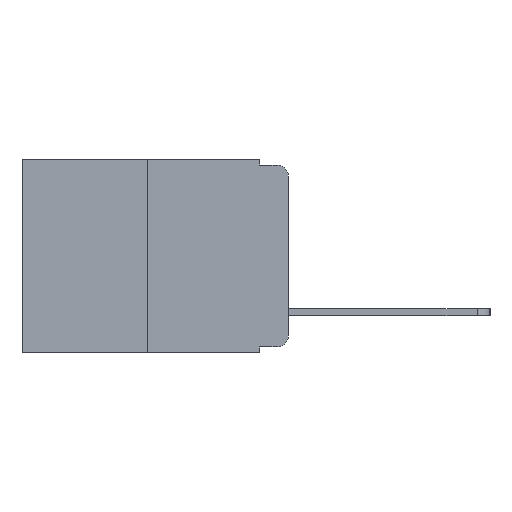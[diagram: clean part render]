
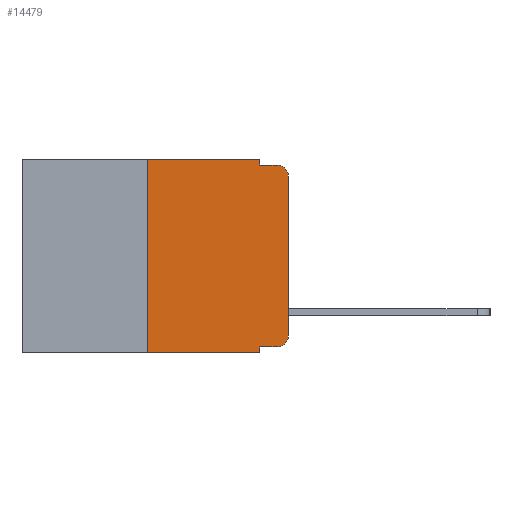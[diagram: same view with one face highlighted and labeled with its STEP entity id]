
A CAD part, left-side view. The second image highlights one B-rep face of the part: STEP entity #14479.
In plain terms, the highlighted planar face has unit normal (-1, 0, 0).
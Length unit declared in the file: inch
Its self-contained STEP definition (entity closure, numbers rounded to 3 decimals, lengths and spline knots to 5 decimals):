
#129 = CARTESIAN_POINT ( 'NONE',  ( 0., 0.02, -0.333 ) ) ;
#312 = CARTESIAN_POINT ( 'NONE',  ( 0., 0.051, 0. ) ) ;
#327 = CARTESIAN_POINT ( 'NONE',  ( 0., 0.02, -0.03 ) ) ;
#511 = FACE_OUTER_BOUND ( 'NONE', #15058, .T. ) ;
#1248 = ORIENTED_EDGE ( 'NONE', *, *, #13304, .T. ) ;
#1250 = DIRECTION ( 'NONE',  ( 0., 0., -1. ) ) ;
#1669 = LINE ( 'NONE', #10075, #18219 ) ;
#2333 = DIRECTION ( 'NONE',  ( 0., 0., -1. ) ) ;
#2387 = VECTOR ( 'NONE', #7106, 39.37008 ) ;
#2648 = CARTESIAN_POINT ( 'NONE',  ( 0., 0.051, 0. ) ) ;
#2941 = EDGE_CURVE ( 'NONE', #19305, #21995, #11428, .T. ) ;
#2993 = LINE ( 'NONE', #20361, #2387 ) ;
#3314 = CARTESIAN_POINT ( 'NONE',  ( 0., 0.051, 0. ) ) ;
#3484 = DIRECTION ( 'NONE',  ( 0., 0., -1. ) ) ;
#3697 = EDGE_CURVE ( 'NONE', #3745, #8694, #10330, .T. ) ;
#3732 = VERTEX_POINT ( 'NONE', #7058 ) ;
#3745 = VERTEX_POINT ( 'NONE', #2648 ) ;
#4067 = CARTESIAN_POINT ( 'NONE',  ( 0., 0.25, -0.343 ) ) ;
#4277 = ORIENTED_EDGE ( 'NONE', *, *, #2941, .T. ) ;
#4304 = VECTOR ( 'NONE', #4906, 39.37008 ) ;
#4624 = ORIENTED_EDGE ( 'NONE', *, *, #7235, .T. ) ;
#4906 = DIRECTION ( 'NONE',  ( 0., -1., 0. ) ) ;
#5001 = DIRECTION ( 'NONE',  ( 0., 0., 1. ) ) ;
#5037 = ORIENTED_EDGE ( 'NONE', *, *, #8382, .T. ) ;
#5169 = ORIENTED_EDGE ( 'NONE', *, *, #20959, .F. ) ;
#5822 = VECTOR ( 'NONE', #3484, 39.37008 ) ;
#5860 = AXIS2_PLACEMENT_3D ( 'NONE', #10078, #11786, #1250 ) ;
#6322 = CARTESIAN_POINT ( 'NONE',  ( 0., 0., -0.313 ) ) ;
#6383 = CARTESIAN_POINT ( 'NONE',  ( 0., 0.051, -0.333 ) ) ;
#6390 = VERTEX_POINT ( 'NONE', #15175 ) ;
#6841 = VERTEX_POINT ( 'NONE', #6383 ) ;
#7058 = CARTESIAN_POINT ( 'NONE',  ( 0., 0.051, -0.343 ) ) ;
#7106 = DIRECTION ( 'NONE',  ( 0., -1., 0. ) ) ;
#7235 = EDGE_CURVE ( 'NONE', #21995, #15967, #21006, .T. ) ;
#8260 = EDGE_CURVE ( 'NONE', #21812, #3732, #20229, .T. ) ;
#8339 = LINE ( 'NONE', #12148, #16635 ) ;
#8382 = EDGE_CURVE ( 'NONE', #15967, #11185, #14354, .T. ) ;
#8426 = PLANE ( 'NONE',  #5860 ) ;
#8650 = ORIENTED_EDGE ( 'NONE', *, *, #3697, .F. ) ;
#8690 = LINE ( 'NONE', #312, #16982 ) ;
#8694 = VERTEX_POINT ( 'NONE', #11718 ) ;
#8819 = EDGE_CURVE ( 'NONE', #6390, #3745, #8339, .T. ) ;
#9137 = ORIENTED_EDGE ( 'NONE', *, *, #8260, .T. ) ;
#10075 = CARTESIAN_POINT ( 'NONE',  ( 0., 0.25, 0. ) ) ;
#10078 = CARTESIAN_POINT ( 'NONE',  ( 0., 0.473, 0. ) ) ;
#10170 = ORIENTED_EDGE ( 'NONE', *, *, #15453, .F. ) ;
#10330 = LINE ( 'NONE', #3314, #5822 ) ;
#10679 = DIRECTION ( 'NONE',  ( 0., -1., 0. ) ) ;
#10696 = DIRECTION ( 'NONE',  ( 0., 0., 1. ) ) ;
#11185 = VERTEX_POINT ( 'NONE', #22221 ) ;
#11428 = CIRCLE ( 'NONE', #12964, 0.02 ) ;
#11494 = ORIENTED_EDGE ( 'NONE', *, *, #8819, .F. ) ;
#11718 = CARTESIAN_POINT ( 'NONE',  ( 0., 0.051, -0.01 ) ) ;
#11750 = VECTOR ( 'NONE', #10696, 39.37008 ) ;
#11772 = DIRECTION ( 'NONE',  ( -1., 0., 0. ) ) ;
#11786 = DIRECTION ( 'NONE',  ( 1., 0., 0. ) ) ;
#11806 = DIRECTION ( 'NONE',  ( 0., 0., -1. ) ) ;
#12148 = CARTESIAN_POINT ( 'NONE',  ( 0., 0.473, 0. ) ) ;
#12699 = DIRECTION ( 'NONE',  ( -1., 0., 0. ) ) ;
#12861 = ORIENTED_EDGE ( 'NONE', *, *, #16568, .F. ) ;
#12932 = CARTESIAN_POINT ( 'NONE',  ( 0., 0.02, -0.313 ) ) ;
#12964 = AXIS2_PLACEMENT_3D ( 'NONE', #12932, #11772, #11806 ) ;
#13304 = EDGE_CURVE ( 'NONE', #6841, #19305, #17697, .T. ) ;
#13383 = CARTESIAN_POINT ( 'NONE',  ( 0., 0.051, -0.333 ) ) ;
#14342 = DIRECTION ( 'NONE',  ( 0., 0., -1. ) ) ;
#14354 = CIRCLE ( 'NONE', #16574, 0.02 ) ;
#14479 = ADVANCED_FACE ( 'NONE', ( #511 ), #8426, .F. ) ;
#15058 = EDGE_LOOP ( 'NONE', ( #4624, #5037, #5169, #8650, #11494, #12861, #9137, #10170, #1248, #4277 ) ) ;
#15175 = CARTESIAN_POINT ( 'NONE',  ( 0., 0.25, 0. ) ) ;
#15453 = EDGE_CURVE ( 'NONE', #6841, #3732, #8690, .T. ) ;
#15847 = VECTOR ( 'NONE', #10679, 39.37008 ) ;
#15967 = VERTEX_POINT ( 'NONE', #19247 ) ;
#16568 = EDGE_CURVE ( 'NONE', #21812, #6390, #1669, .T. ) ;
#16574 = AXIS2_PLACEMENT_3D ( 'NONE', #327, #12699, #2333 ) ;
#16635 = VECTOR ( 'NONE', #18680, 39.37008 ) ;
#16982 = VECTOR ( 'NONE', #14342, 39.37008 ) ;
#17697 = LINE ( 'NONE', #13383, #4304 ) ;
#18219 = VECTOR ( 'NONE', #5001, 39.37008 ) ;
#18680 = DIRECTION ( 'NONE',  ( 0., -1., 0. ) ) ;
#19247 = CARTESIAN_POINT ( 'NONE',  ( 0., 0., -0.03 ) ) ;
#19305 = VERTEX_POINT ( 'NONE', #129 ) ;
#20229 = LINE ( 'NONE', #22148, #15847 ) ;
#20361 = CARTESIAN_POINT ( 'NONE',  ( 0., 0.051, -0.01 ) ) ;
#20578 = CARTESIAN_POINT ( 'NONE',  ( 0., 0., 0. ) ) ;
#20959 = EDGE_CURVE ( 'NONE', #8694, #11185, #2993, .T. ) ;
#21006 = LINE ( 'NONE', #20578, #11750 ) ;
#21812 = VERTEX_POINT ( 'NONE', #4067 ) ;
#21995 = VERTEX_POINT ( 'NONE', #6322 ) ;
#22148 = CARTESIAN_POINT ( 'NONE',  ( 0., 0.473, -0.343 ) ) ;
#22221 = CARTESIAN_POINT ( 'NONE',  ( 0., 0.02, -0.01 ) ) ;
